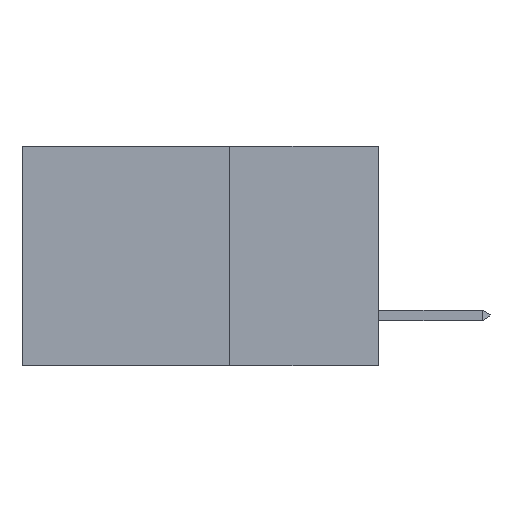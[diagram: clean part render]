
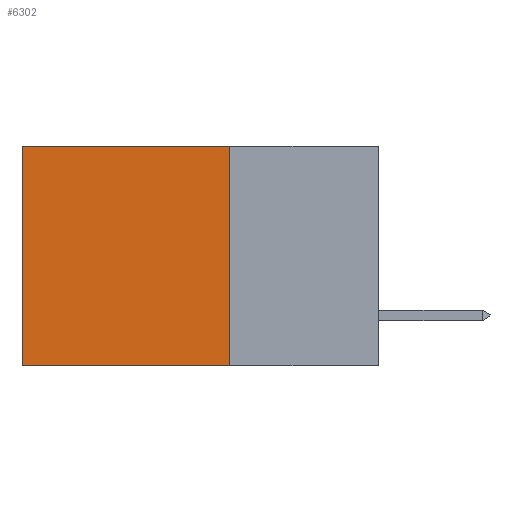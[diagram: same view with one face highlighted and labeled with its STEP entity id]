
A CAD part, left-side view. The second image highlights one B-rep face of the part: STEP entity #6302.
In plain terms, the highlighted planar face has unit normal (-1, 0, 0).
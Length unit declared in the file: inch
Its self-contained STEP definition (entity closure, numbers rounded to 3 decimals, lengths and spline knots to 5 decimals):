
#490 = DIRECTION ( 'NONE',  ( 0., 0., -1. ) ) ;
#1055 = DIRECTION ( 'NONE',  ( 0., 0., -1. ) ) ;
#1488 = EDGE_LOOP ( 'NONE', ( #24574, #23389, #16038, #2158 ) ) ;
#1983 = CARTESIAN_POINT ( 'NONE',  ( 0.2615, 0.25, 0. ) ) ;
#2158 = ORIENTED_EDGE ( 'NONE', *, *, #14138, .T. ) ;
#3179 = AXIS2_PLACEMENT_3D ( 'NONE', #9515, #23242, #5443 ) ;
#4158 = LINE ( 'NONE', #6119, #15169 ) ;
#5443 = DIRECTION ( 'NONE',  ( 0., 0., -1. ) ) ;
#6052 = VECTOR ( 'NONE', #18411, 39.37008 ) ;
#6119 = CARTESIAN_POINT ( 'NONE',  ( 0.2615, 0.25, -0.37 ) ) ;
#6130 = EDGE_CURVE ( 'NONE', #20206, #7387, #18289, .T. ) ;
#6302 = ADVANCED_FACE ( 'NONE', ( #15499 ), #21390, .F. ) ;
#7387 = VERTEX_POINT ( 'NONE', #16497 ) ;
#9515 = CARTESIAN_POINT ( 'NONE',  ( 0.2615, 0.25, -0.37 ) ) ;
#9802 = VECTOR ( 'NONE', #1055, 39.37008 ) ;
#10268 = VERTEX_POINT ( 'NONE', #11426 ) ;
#10452 = CARTESIAN_POINT ( 'NONE',  ( 0.2615, 0.25, -0.37 ) ) ;
#11426 = CARTESIAN_POINT ( 'NONE',  ( 0.2615, 0.6, 0. ) ) ;
#13196 = LINE ( 'NONE', #23002, #9802 ) ;
#14138 = EDGE_CURVE ( 'NONE', #20595, #10268, #14497, .T. ) ;
#14497 = LINE ( 'NONE', #1983, #20151 ) ;
#14601 = EDGE_CURVE ( 'NONE', #20595, #20206, #4158, .T. ) ;
#14954 = CARTESIAN_POINT ( 'NONE',  ( 0.2615, 0.25, -0.37 ) ) ;
#15169 = VECTOR ( 'NONE', #490, 39.37008 ) ;
#15499 = FACE_OUTER_BOUND ( 'NONE', #1488, .T. ) ;
#15649 = EDGE_CURVE ( 'NONE', #10268, #7387, #13196, .T. ) ;
#16038 = ORIENTED_EDGE ( 'NONE', *, *, #14601, .F. ) ;
#16497 = CARTESIAN_POINT ( 'NONE',  ( 0.2615, 0.6, -0.37 ) ) ;
#18157 = DIRECTION ( 'NONE',  ( 0., 1., 0. ) ) ;
#18289 = LINE ( 'NONE', #10452, #6052 ) ;
#18411 = DIRECTION ( 'NONE',  ( 0., 1., 0. ) ) ;
#19778 = CARTESIAN_POINT ( 'NONE',  ( 0.2615, 0.25, 0. ) ) ;
#20151 = VECTOR ( 'NONE', #18157, 39.37008 ) ;
#20206 = VERTEX_POINT ( 'NONE', #14954 ) ;
#20595 = VERTEX_POINT ( 'NONE', #19778 ) ;
#21390 = PLANE ( 'NONE',  #3179 ) ;
#23002 = CARTESIAN_POINT ( 'NONE',  ( 0.2615, 0.6, -0.37 ) ) ;
#23242 = DIRECTION ( 'NONE',  ( 1., 0., 0. ) ) ;
#23389 = ORIENTED_EDGE ( 'NONE', *, *, #6130, .F. ) ;
#24574 = ORIENTED_EDGE ( 'NONE', *, *, #15649, .T. ) ;
